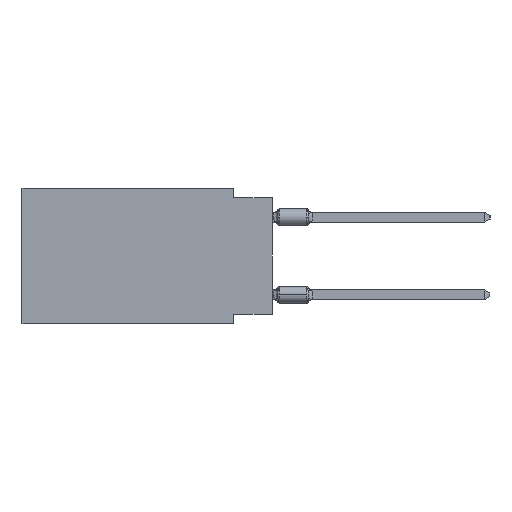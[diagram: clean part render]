
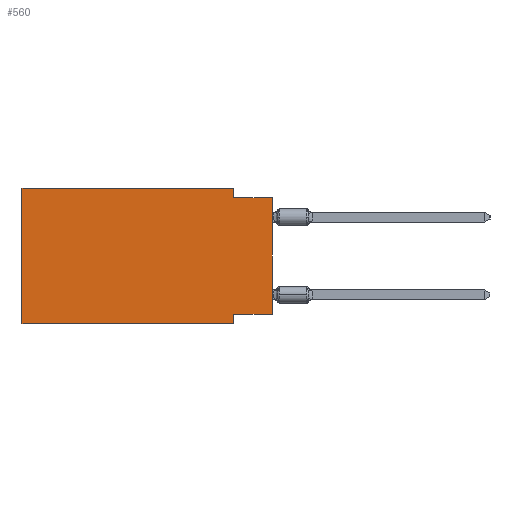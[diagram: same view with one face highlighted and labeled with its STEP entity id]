
A CAD part, left-side view. The second image highlights one B-rep face of the part: STEP entity #560.
In plain terms, the highlighted planar face has unit normal (-1, 0, 0).
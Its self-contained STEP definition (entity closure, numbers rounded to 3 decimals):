
#560 = ADVANCED_FACE ( 'NONE', ( #4355 ), #6389, .F. ) ;
#1008 = CARTESIAN_POINT ( 'NONE',  ( 0., 2.54, 0. ) ) ;
#1122 = CARTESIAN_POINT ( 'NONE',  ( 0., 0., -8.255 ) ) ;
#1360 = VECTOR ( 'NONE', #4630, 1000. ) ;
#1763 = DIRECTION ( 'NONE',  ( 0., -1., 0. ) ) ;
#2570 = CARTESIAN_POINT ( 'NONE',  ( 0., 0., -8.255 ) ) ;
#3194 = VECTOR ( 'NONE', #29656, 1000. ) ;
#3907 = EDGE_CURVE ( 'NONE', #11672, #4522, #18060, .T. ) ;
#4015 = EDGE_CURVE ( 'NONE', #19004, #4522, #16032, .T. ) ;
#4132 = ORIENTED_EDGE ( 'NONE', *, *, #30105, .F. ) ;
#4135 = CARTESIAN_POINT ( 'NONE',  ( 0., 2.54, 0. ) ) ;
#4221 = VECTOR ( 'NONE', #18481, 1000. ) ;
#4355 = FACE_OUTER_BOUND ( 'NONE', #13775, .T. ) ;
#4522 = VERTEX_POINT ( 'NONE', #12154 ) ;
#4630 = DIRECTION ( 'NONE',  ( 0., 1., 0. ) ) ;
#4894 = CARTESIAN_POINT ( 'NONE',  ( 0., 2.54, -8.89 ) ) ;
#4959 = CARTESIAN_POINT ( 'NONE',  ( 0., 2.54, -8.89 ) ) ;
#5729 = VECTOR ( 'NONE', #1763, 1000. ) ;
#5760 = ORIENTED_EDGE ( 'NONE', *, *, #30792, .F. ) ;
#6389 = PLANE ( 'NONE',  #30424 ) ;
#6523 = EDGE_CURVE ( 'NONE', #11672, #27553, #28598, .T. ) ;
#7900 = DIRECTION ( 'NONE',  ( 0., -1., 0. ) ) ;
#8106 = ORIENTED_EDGE ( 'NONE', *, *, #4015, .F. ) ;
#8361 = CARTESIAN_POINT ( 'NONE',  ( 0., 0., 0. ) ) ;
#8386 = DIRECTION ( 'NONE',  ( 0., 0., -1. ) ) ;
#8600 = VERTEX_POINT ( 'NONE', #15056 ) ;
#10033 = CARTESIAN_POINT ( 'NONE',  ( 0., 16.383, 0. ) ) ;
#11407 = DIRECTION ( 'NONE',  ( 0., 0., -1. ) ) ;
#11672 = VERTEX_POINT ( 'NONE', #1122 ) ;
#12154 = CARTESIAN_POINT ( 'NONE',  ( 0., 0., -0.635 ) ) ;
#12376 = ORIENTED_EDGE ( 'NONE', *, *, #3907, .T. ) ;
#12467 = VERTEX_POINT ( 'NONE', #4135 ) ;
#13547 = CARTESIAN_POINT ( 'NONE',  ( 0., 16.383, 0. ) ) ;
#13739 = CARTESIAN_POINT ( 'NONE',  ( 0., 16.383, 0. ) ) ;
#13775 = EDGE_LOOP ( 'NONE', ( #12376, #8106, #4132, #27718, #23527, #19774, #5760, #14110 ) ) ;
#14110 = ORIENTED_EDGE ( 'NONE', *, *, #6523, .F. ) ;
#14452 = DIRECTION ( 'NONE',  ( 0., 0., -1. ) ) ;
#14633 = EDGE_CURVE ( 'NONE', #22881, #12467, #17707, .T. ) ;
#14753 = VECTOR ( 'NONE', #14452, 1000. ) ;
#15056 = CARTESIAN_POINT ( 'NONE',  ( 0., 16.383, -8.89 ) ) ;
#15664 = CARTESIAN_POINT ( 'NONE',  ( 0., 16.383, 0. ) ) ;
#16032 = LINE ( 'NONE', #25733, #5729 ) ;
#16949 = CARTESIAN_POINT ( 'NONE',  ( 0., 2.54, -8.255 ) ) ;
#17707 = LINE ( 'NONE', #10033, #21348 ) ;
#17764 = CARTESIAN_POINT ( 'NONE',  ( 0., 16.383, -8.89 ) ) ;
#17932 = LINE ( 'NONE', #17764, #30230 ) ;
#18060 = LINE ( 'NONE', #8361, #3194 ) ;
#18481 = DIRECTION ( 'NONE',  ( 0., 0., 1. ) ) ;
#19004 = VERTEX_POINT ( 'NONE', #30499 ) ;
#19774 = ORIENTED_EDGE ( 'NONE', *, *, #28940, .T. ) ;
#20813 = DIRECTION ( 'NONE',  ( 1., 0., 0. ) ) ;
#21348 = VECTOR ( 'NONE', #29151, 1000. ) ;
#22881 = VERTEX_POINT ( 'NONE', #13547 ) ;
#23027 = LINE ( 'NONE', #15664, #4221 ) ;
#23527 = ORIENTED_EDGE ( 'NONE', *, *, #25702, .F. ) ;
#24755 = VECTOR ( 'NONE', #8386, 1000. ) ;
#25702 = EDGE_CURVE ( 'NONE', #8600, #22881, #23027, .T. ) ;
#25733 = CARTESIAN_POINT ( 'NONE',  ( 0., 0., -0.635 ) ) ;
#26502 = LINE ( 'NONE', #4894, #14753 ) ;
#27161 = LINE ( 'NONE', #1008, #24755 ) ;
#27553 = VERTEX_POINT ( 'NONE', #16949 ) ;
#27718 = ORIENTED_EDGE ( 'NONE', *, *, #14633, .F. ) ;
#28418 = VERTEX_POINT ( 'NONE', #4959 ) ;
#28598 = LINE ( 'NONE', #2570, #1360 ) ;
#28940 = EDGE_CURVE ( 'NONE', #8600, #28418, #17932, .T. ) ;
#29151 = DIRECTION ( 'NONE',  ( 0., -1., 0. ) ) ;
#29656 = DIRECTION ( 'NONE',  ( 0., 0., 1. ) ) ;
#30105 = EDGE_CURVE ( 'NONE', #12467, #19004, #27161, .T. ) ;
#30230 = VECTOR ( 'NONE', #7900, 1000. ) ;
#30424 = AXIS2_PLACEMENT_3D ( 'NONE', #13739, #20813, #11407 ) ;
#30499 = CARTESIAN_POINT ( 'NONE',  ( 0., 2.54, -0.635 ) ) ;
#30792 = EDGE_CURVE ( 'NONE', #27553, #28418, #26502, .T. ) ;
